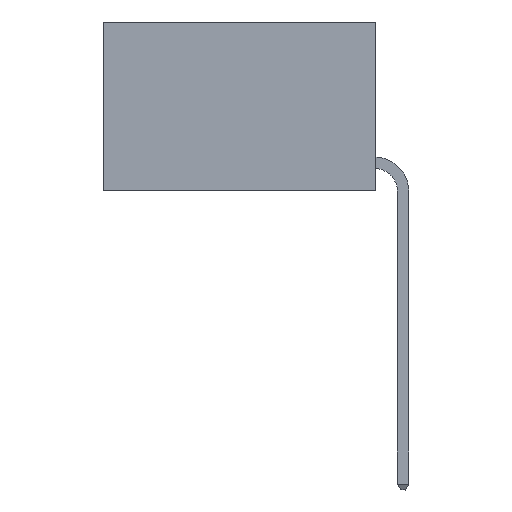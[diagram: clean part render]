
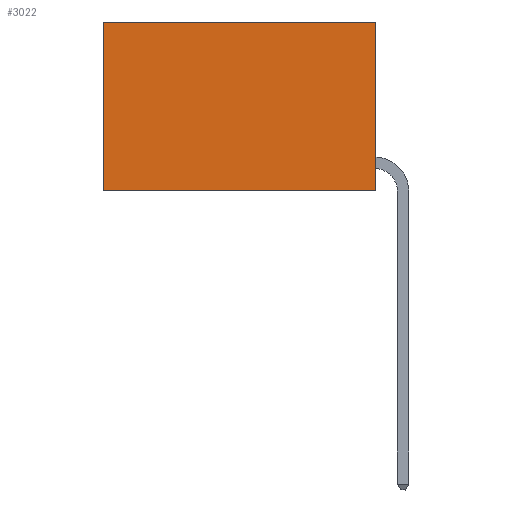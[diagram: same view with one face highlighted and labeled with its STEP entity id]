
A CAD part, left-side view. The second image highlights one B-rep face of the part: STEP entity #3022.
In plain terms, the highlighted planar face has unit normal (-1, 0, 0).
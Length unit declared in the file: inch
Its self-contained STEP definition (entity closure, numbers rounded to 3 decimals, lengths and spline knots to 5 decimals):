
#37 = VECTOR ( 'NONE', #15055, 39.37008 ) ;
#73 = EDGE_CURVE ( 'NONE', #13107, #6436, #12380, .T. ) ;
#457 = EDGE_CURVE ( 'NONE', #6436, #13801, #3747, .T. ) ;
#1167 = CARTESIAN_POINT ( 'NONE',  ( 0.2625, 0., 0. ) ) ;
#2006 = FACE_OUTER_BOUND ( 'NONE', #10856, .T. ) ;
#2269 = DIRECTION ( 'NONE',  ( 1., 0., 0. ) ) ;
#3021 = VECTOR ( 'NONE', #3488, 39.37008 ) ;
#3022 = ADVANCED_FACE ( 'NONE', ( #2006 ), #9335, .F. ) ;
#3211 = LINE ( 'NONE', #12851, #37 ) ;
#3488 = DIRECTION ( 'NONE',  ( 0., 1., 0. ) ) ;
#3747 = LINE ( 'NONE', #13400, #9627 ) ;
#4335 = CARTESIAN_POINT ( 'NONE',  ( 0.2625, 0.6, 0. ) ) ;
#5913 = AXIS2_PLACEMENT_3D ( 'NONE', #13944, #2269, #10508 ) ;
#5973 = ORIENTED_EDGE ( 'NONE', *, *, #457, .T. ) ;
#6436 = VERTEX_POINT ( 'NONE', #4335 ) ;
#8047 = ORIENTED_EDGE ( 'NONE', *, *, #73, .T. ) ;
#8491 = DIRECTION ( 'NONE',  ( 0., 1., 0. ) ) ;
#8621 = VECTOR ( 'NONE', #8491, 39.37008 ) ;
#8746 = ORIENTED_EDGE ( 'NONE', *, *, #12745, .F. ) ;
#9106 = CARTESIAN_POINT ( 'NONE',  ( 0.2625, 0., 0. ) ) ;
#9335 = PLANE ( 'NONE',  #5913 ) ;
#9627 = VECTOR ( 'NONE', #14284, 39.37008 ) ;
#9894 = CARTESIAN_POINT ( 'NONE',  ( 0.2625, 0.6, -0.37 ) ) ;
#10508 = DIRECTION ( 'NONE',  ( 0., 0., -1. ) ) ;
#10856 = EDGE_LOOP ( 'NONE', ( #5973, #8746, #11852, #8047 ) ) ;
#11852 = ORIENTED_EDGE ( 'NONE', *, *, #14768, .F. ) ;
#12096 = LINE ( 'NONE', #14273, #8621 ) ;
#12195 = VERTEX_POINT ( 'NONE', #13374 ) ;
#12380 = LINE ( 'NONE', #1167, #3021 ) ;
#12745 = EDGE_CURVE ( 'NONE', #12195, #13801, #12096, .T. ) ;
#12851 = CARTESIAN_POINT ( 'NONE',  ( 0.2625, 0., 0. ) ) ;
#13107 = VERTEX_POINT ( 'NONE', #9106 ) ;
#13374 = CARTESIAN_POINT ( 'NONE',  ( 0.2625, 0., -0.37 ) ) ;
#13400 = CARTESIAN_POINT ( 'NONE',  ( 0.2625, 0.6, 0. ) ) ;
#13801 = VERTEX_POINT ( 'NONE', #9894 ) ;
#13944 = CARTESIAN_POINT ( 'NONE',  ( 0.2625, 0., 0. ) ) ;
#14273 = CARTESIAN_POINT ( 'NONE',  ( 0.2625, 0., -0.37 ) ) ;
#14284 = DIRECTION ( 'NONE',  ( 0., 0., -1. ) ) ;
#14768 = EDGE_CURVE ( 'NONE', #13107, #12195, #3211, .T. ) ;
#15055 = DIRECTION ( 'NONE',  ( 0., 0., -1. ) ) ;
